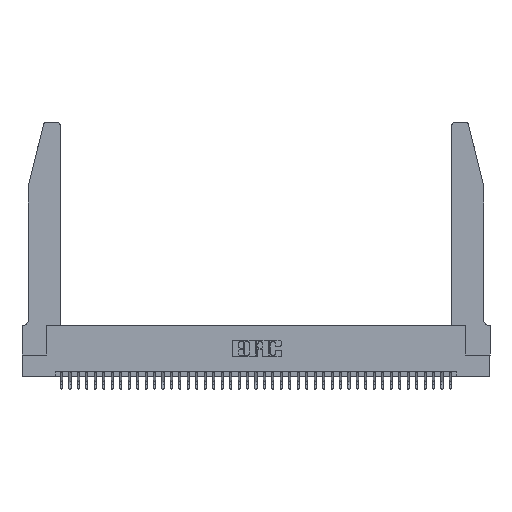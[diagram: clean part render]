
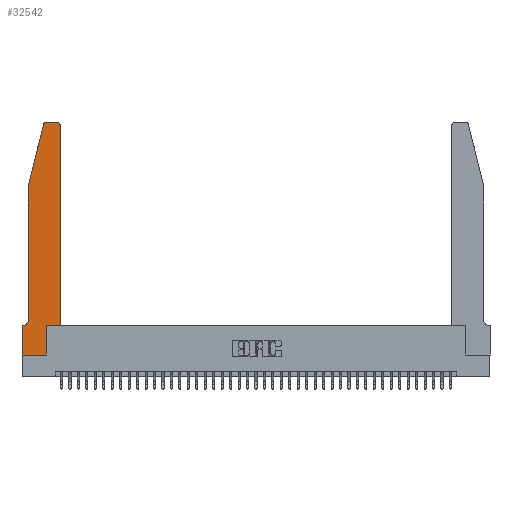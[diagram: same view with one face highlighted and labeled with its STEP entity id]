
A CAD part, top view. The second image highlights one B-rep face of the part: STEP entity #32542.
In plain terms, the highlighted planar face has unit normal (0, 0, 1).
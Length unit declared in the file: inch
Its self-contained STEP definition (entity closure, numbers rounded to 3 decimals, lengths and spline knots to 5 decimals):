
#460 = CARTESIAN_POINT ( 'NONE',  ( 0., 0., 0.37 ) ) ;
#654 = CARTESIAN_POINT ( 'NONE',  ( 0.0755, 0.35, 0.37 ) ) ;
#696 = CARTESIAN_POINT ( 'NONE',  ( 0.284, 2.72, 0.37 ) ) ;
#996 = DIRECTION ( 'NONE',  ( 0., -1., 0. ) ) ;
#1110 = DIRECTION ( 'NONE',  ( 0., 0., 1. ) ) ;
#1801 = VERTEX_POINT ( 'NONE', #8226 ) ;
#2125 = VECTOR ( 'NONE', #996, 39.37008 ) ;
#2925 = CARTESIAN_POINT ( 'NONE',  ( 0., 0., 0.37 ) ) ;
#4022 = DIRECTION ( 'NONE',  ( -1., 0., 0. ) ) ;
#4211 = LINE ( 'NONE', #460, #37042 ) ;
#5089 = EDGE_CURVE ( 'NONE', #11027, #36946, #41179, .T. ) ;
#5417 = AXIS2_PLACEMENT_3D ( 'NONE', #13014, #16214, #19426 ) ;
#6116 = VERTEX_POINT ( 'NONE', #21487 ) ;
#6536 = VERTEX_POINT ( 'NONE', #14421 ) ;
#6869 = AXIS2_PLACEMENT_3D ( 'NONE', #696, #38689, #13434 ) ;
#6958 = VERTEX_POINT ( 'NONE', #10015 ) ;
#7320 = VERTEX_POINT ( 'NONE', #15440 ) ;
#7506 = ORIENTED_EDGE ( 'NONE', *, *, #9410, .T. ) ;
#7600 = LINE ( 'NONE', #654, #23550 ) ;
#7671 = CIRCLE ( 'NONE', #37800, 0.03 ) ;
#7785 = VERTEX_POINT ( 'NONE', #33585 ) ;
#7837 = CARTESIAN_POINT ( 'NONE',  ( 0., 0.35, 0.37 ) ) ;
#8096 = EDGE_CURVE ( 'NONE', #36946, #6116, #38466, .T. ) ;
#8226 = CARTESIAN_POINT ( 'NONE',  ( 0.0055, 0.35, 0.37 ) ) ;
#8248 = EDGE_CURVE ( 'NONE', #6958, #32406, #12650, .T. ) ;
#8541 = CARTESIAN_POINT ( 'NONE',  ( 0.284, 2.75, 0.37 ) ) ;
#8813 = DIRECTION ( 'NONE',  ( 1., 0., 0. ) ) ;
#9410 = EDGE_CURVE ( 'NONE', #21045, #1801, #24043, .T. ) ;
#9420 = ORIENTED_EDGE ( 'NONE', *, *, #5089, .T. ) ;
#10015 = CARTESIAN_POINT ( 'NONE',  ( 0.2865, 0., 0.37 ) ) ;
#10754 = PLANE ( 'NONE',  #33462 ) ;
#10882 = ORIENTED_EDGE ( 'NONE', *, *, #8248, .T. ) ;
#11027 = VERTEX_POINT ( 'NONE', #8541 ) ;
#11063 = EDGE_LOOP ( 'NONE', ( #17086, #9420, #12783, #21946, #7506, #13626, #38581, #33183, #10882, #38921, #34813, #13447 ) ) ;
#12144 = EDGE_CURVE ( 'NONE', #6536, #30622, #22325, .T. ) ;
#12166 = DIRECTION ( 'NONE',  ( 0., 0., 1. ) ) ;
#12650 = LINE ( 'NONE', #40043, #14183 ) ;
#12783 = ORIENTED_EDGE ( 'NONE', *, *, #8096, .T. ) ;
#13014 = CARTESIAN_POINT ( 'NONE',  ( 0.0055, 0.42, 0.37 ) ) ;
#13434 = DIRECTION ( 'NONE',  ( 1., 0., 0. ) ) ;
#13447 = ORIENTED_EDGE ( 'NONE', *, *, #39327, .T. ) ;
#13580 = EDGE_CURVE ( 'NONE', #30622, #6958, #4211, .T. ) ;
#13626 = ORIENTED_EDGE ( 'NONE', *, *, #28483, .T. ) ;
#13728 = CARTESIAN_POINT ( 'NONE',  ( 0.0755, 2., 0.37 ) ) ;
#14143 = LINE ( 'NONE', #26509, #2125 ) ;
#14183 = VECTOR ( 'NONE', #40188, 39.37008 ) ;
#14421 = CARTESIAN_POINT ( 'NONE',  ( 0., 0.35, 0.37 ) ) ;
#14449 = CARTESIAN_POINT ( 'NONE',  ( 0.0755, 0.42, 0.37 ) ) ;
#15440 = CARTESIAN_POINT ( 'NONE',  ( 0.4505, 0.35, 0.37 ) ) ;
#16214 = DIRECTION ( 'NONE',  ( 0., 0., -1. ) ) ;
#16469 = CARTESIAN_POINT ( 'NONE',  ( 0.4505, 2.72, 0.37 ) ) ;
#17086 = ORIENTED_EDGE ( 'NONE', *, *, #36330, .T. ) ;
#19426 = DIRECTION ( 'NONE',  ( -1., 0., 0. ) ) ;
#19669 = CARTESIAN_POINT ( 'NONE',  ( 0.2865, 0.35, 0.37 ) ) ;
#19760 = VECTOR ( 'NONE', #8813, 39.37008 ) ;
#20103 = DIRECTION ( 'NONE',  ( 1., 0., 0. ) ) ;
#20130 = DIRECTION ( 'NONE',  ( -0.239, -0.971, 0. ) ) ;
#20531 = CARTESIAN_POINT ( 'NONE',  ( 0.4505, 0.35, 0.37 ) ) ;
#20855 = CARTESIAN_POINT ( 'NONE',  ( 0.4505, 0.35, 0.37 ) ) ;
#21045 = VERTEX_POINT ( 'NONE', #14449 ) ;
#21487 = CARTESIAN_POINT ( 'NONE',  ( 0.0755, 2., 0.37 ) ) ;
#21946 = ORIENTED_EDGE ( 'NONE', *, *, #27874, .T. ) ;
#22277 = FACE_OUTER_BOUND ( 'NONE', #11063, .T. ) ;
#22325 = LINE ( 'NONE', #2925, #29209 ) ;
#22390 = VECTOR ( 'NONE', #32868, 39.37008 ) ;
#22818 = DIRECTION ( 'NONE',  ( 1., 0., 0. ) ) ;
#23550 = VECTOR ( 'NONE', #4022, 39.37008 ) ;
#23667 = CARTESIAN_POINT ( 'NONE',  ( 0., 0., 0.37 ) ) ;
#24043 = CIRCLE ( 'NONE', #5417, 0.07 ) ;
#24299 = DIRECTION ( 'NONE',  ( 0., 1., 0. ) ) ;
#25009 = LINE ( 'NONE', #20855, #27499 ) ;
#25072 = DIRECTION ( 'NONE',  ( 0., -1., 0. ) ) ;
#25729 = LINE ( 'NONE', #20531, #19760 ) ;
#26509 = CARTESIAN_POINT ( 'NONE',  ( 0.0755, 2., 0.37 ) ) ;
#27499 = VECTOR ( 'NONE', #24299, 39.37008 ) ;
#27874 = EDGE_CURVE ( 'NONE', #6116, #21045, #14143, .T. ) ;
#28483 = EDGE_CURVE ( 'NONE', #1801, #6536, #7600, .T. ) ;
#29209 = VECTOR ( 'NONE', #25072, 39.37008 ) ;
#29889 = EDGE_CURVE ( 'NONE', #32406, #7320, #25729, .T. ) ;
#30622 = VERTEX_POINT ( 'NONE', #23667 ) ;
#32396 = VERTEX_POINT ( 'NONE', #16469 ) ;
#32406 = VERTEX_POINT ( 'NONE', #19669 ) ;
#32542 = ADVANCED_FACE ( 'NONE', ( #22277 ), #10754, .T. ) ;
#32868 = DIRECTION ( 'NONE',  ( -1., 0., 0. ) ) ;
#33183 = ORIENTED_EDGE ( 'NONE', *, *, #13580, .T. ) ;
#33462 = AXIS2_PLACEMENT_3D ( 'NONE', #7837, #1110, #20103 ) ;
#33585 = CARTESIAN_POINT ( 'NONE',  ( 0.4205, 2.75, 0.37 ) ) ;
#34383 = DIRECTION ( 'NONE',  ( 1., 0., 0. ) ) ;
#34813 = ORIENTED_EDGE ( 'NONE', *, *, #40306, .T. ) ;
#36258 = LINE ( 'NONE', #36483, #22390 ) ;
#36330 = EDGE_CURVE ( 'NONE', #7785, #11027, #36258, .T. ) ;
#36483 = CARTESIAN_POINT ( 'NONE',  ( 0.2605, 2.75, 0.37 ) ) ;
#36946 = VERTEX_POINT ( 'NONE', #40411 ) ;
#37042 = VECTOR ( 'NONE', #22818, 39.37008 ) ;
#37438 = VECTOR ( 'NONE', #20130, 39.37008 ) ;
#37800 = AXIS2_PLACEMENT_3D ( 'NONE', #40500, #12166, #34383 ) ;
#38466 = LINE ( 'NONE', #13728, #37438 ) ;
#38581 = ORIENTED_EDGE ( 'NONE', *, *, #12144, .T. ) ;
#38689 = DIRECTION ( 'NONE',  ( 0., 0., 1. ) ) ;
#38921 = ORIENTED_EDGE ( 'NONE', *, *, #29889, .T. ) ;
#39327 = EDGE_CURVE ( 'NONE', #32396, #7785, #7671, .T. ) ;
#40043 = CARTESIAN_POINT ( 'NONE',  ( 0.2865, 0.35, 0.37 ) ) ;
#40188 = DIRECTION ( 'NONE',  ( 0., 1., 0. ) ) ;
#40306 = EDGE_CURVE ( 'NONE', #7320, #32396, #25009, .T. ) ;
#40411 = CARTESIAN_POINT ( 'NONE',  ( 0.25487, 2.72718, 0.37 ) ) ;
#40500 = CARTESIAN_POINT ( 'NONE',  ( 0.4205, 2.72, 0.37 ) ) ;
#41179 = CIRCLE ( 'NONE', #6869, 0.03 ) ;
